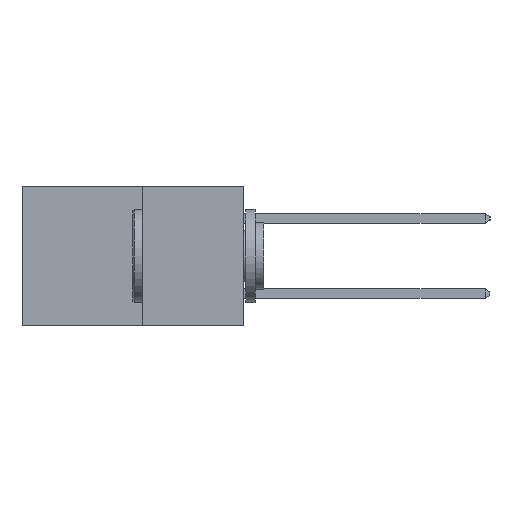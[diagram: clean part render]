
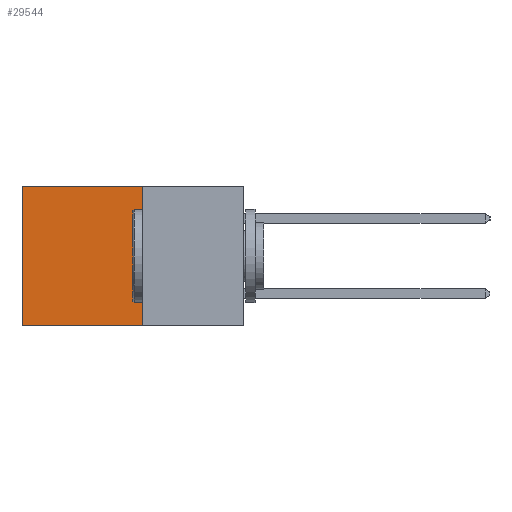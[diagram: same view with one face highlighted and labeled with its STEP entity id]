
A CAD part, left-side view. The second image highlights one B-rep face of the part: STEP entity #29544.
In plain terms, the highlighted planar face has unit normal (-1, 0, 0).
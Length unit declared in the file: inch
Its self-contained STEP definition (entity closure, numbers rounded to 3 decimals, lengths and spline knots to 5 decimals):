
#842 = VERTEX_POINT ( 'NONE', #8535 ) ;
#1989 = DIRECTION ( 'NONE',  ( 0., 0., -1. ) ) ;
#2399 = CARTESIAN_POINT ( 'NONE',  ( 0.277, 0.59, 0. ) ) ;
#2613 = VERTEX_POINT ( 'NONE', #17715 ) ;
#2695 = DIRECTION ( 'NONE',  ( 0., 1., 0. ) ) ;
#2768 = FACE_OUTER_BOUND ( 'NONE', #18142, .T. ) ;
#3122 = CARTESIAN_POINT ( 'NONE',  ( 0.277, 0.27, 0. ) ) ;
#4223 = EDGE_CURVE ( 'NONE', #17558, #22086, #12626, .T. ) ;
#4256 = CARTESIAN_POINT ( 'NONE',  ( 0.277, 0.27, -0.37 ) ) ;
#4331 = ORIENTED_EDGE ( 'NONE', *, *, #15557, .F. ) ;
#4936 = VECTOR ( 'NONE', #7822, 39.37008 ) ;
#6092 = ORIENTED_EDGE ( 'NONE', *, *, #29895, .F. ) ;
#6610 = DIRECTION ( 'NONE',  ( 0., 0., -1. ) ) ;
#7325 = VECTOR ( 'NONE', #6610, 39.37008 ) ;
#7822 = DIRECTION ( 'NONE',  ( 0., 1., 0. ) ) ;
#8535 = CARTESIAN_POINT ( 'NONE',  ( 0.277, 0.59, -0.37 ) ) ;
#9366 = DIRECTION ( 'NONE',  ( 0., 0., -1. ) ) ;
#9415 = ORIENTED_EDGE ( 'NONE', *, *, #4223, .T. ) ;
#10163 = AXIS2_PLACEMENT_3D ( 'NONE', #13741, #16064, #1989 ) ;
#12626 = LINE ( 'NONE', #3122, #23509 ) ;
#13741 = CARTESIAN_POINT ( 'NONE',  ( 0.277, 0.27, -0.37 ) ) ;
#15552 = VECTOR ( 'NONE', #9366, 39.37008 ) ;
#15557 = EDGE_CURVE ( 'NONE', #17558, #2613, #16523, .T. ) ;
#16064 = DIRECTION ( 'NONE',  ( 1., 0., 0. ) ) ;
#16523 = LINE ( 'NONE', #4256, #7325 ) ;
#17558 = VERTEX_POINT ( 'NONE', #24131 ) ;
#17715 = CARTESIAN_POINT ( 'NONE',  ( 0.277, 0.27, -0.37 ) ) ;
#18142 = EDGE_LOOP ( 'NONE', ( #29510, #6092, #4331, #9415 ) ) ;
#20714 = EDGE_CURVE ( 'NONE', #22086, #842, #21723, .T. ) ;
#21000 = CARTESIAN_POINT ( 'NONE',  ( 0.277, 0.59, -0.37 ) ) ;
#21723 = LINE ( 'NONE', #21000, #15552 ) ;
#21834 = CARTESIAN_POINT ( 'NONE',  ( 0.277, 0.27, -0.37 ) ) ;
#22086 = VERTEX_POINT ( 'NONE', #2399 ) ;
#23509 = VECTOR ( 'NONE', #2695, 39.37008 ) ;
#24131 = CARTESIAN_POINT ( 'NONE',  ( 0.277, 0.27, 0. ) ) ;
#29011 = LINE ( 'NONE', #21834, #4936 ) ;
#29510 = ORIENTED_EDGE ( 'NONE', *, *, #20714, .T. ) ;
#29544 = ADVANCED_FACE ( 'NONE', ( #2768 ), #29812, .F. ) ;
#29812 = PLANE ( 'NONE',  #10163 ) ;
#29895 = EDGE_CURVE ( 'NONE', #2613, #842, #29011, .T. ) ;
